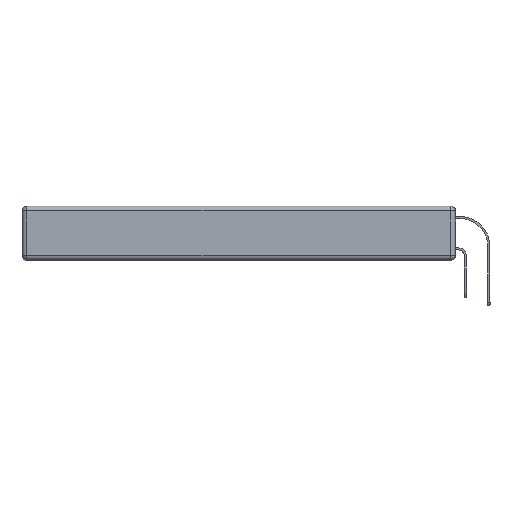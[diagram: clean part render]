
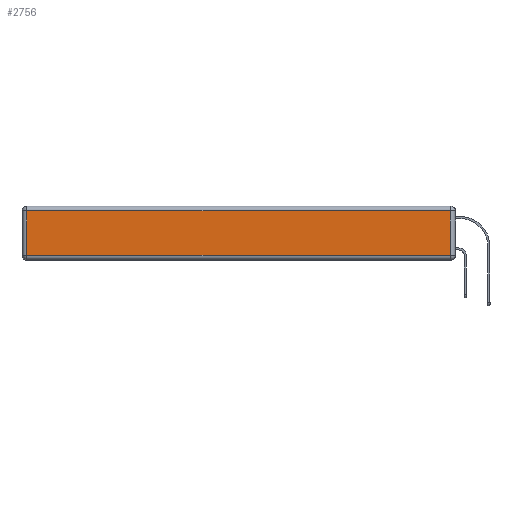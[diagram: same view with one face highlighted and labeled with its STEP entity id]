
A CAD part, left-side view. The second image highlights one B-rep face of the part: STEP entity #2756.
In plain terms, the highlighted planar face has unit normal (-1, 0, 0).
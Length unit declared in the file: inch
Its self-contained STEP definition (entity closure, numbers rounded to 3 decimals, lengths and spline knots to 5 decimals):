
#526 = ORIENTED_EDGE ( 'NONE', *, *, #12476, .T. ) ;
#814 = LINE ( 'NONE', #9463, #4873 ) ;
#867 = VECTOR ( 'NONE', #3666, 39.37008 ) ;
#1168 = CARTESIAN_POINT ( 'NONE',  ( 0., 2.72, -0.03 ) ) ;
#1239 = VERTEX_POINT ( 'NONE', #5424 ) ;
#1809 = CARTESIAN_POINT ( 'NONE',  ( 0., 0., -0.343 ) ) ;
#1946 = DIRECTION ( 'NONE',  ( 0., 0., 1. ) ) ;
#2121 = LINE ( 'NONE', #9834, #4508 ) ;
#2756 = ADVANCED_FACE ( 'NONE', ( #10301 ), #12660, .T. ) ;
#2794 = EDGE_CURVE ( 'NONE', #1239, #9489, #814, .T. ) ;
#2944 = DIRECTION ( 'NONE',  ( -1., 0., 0. ) ) ;
#3602 = CARTESIAN_POINT ( 'NONE',  ( 0., 0., -0.313 ) ) ;
#3666 = DIRECTION ( 'NONE',  ( 0., -1., 0. ) ) ;
#4508 = VECTOR ( 'NONE', #9770, 39.37008 ) ;
#4873 = VECTOR ( 'NONE', #13863, 39.37008 ) ;
#5424 = CARTESIAN_POINT ( 'NONE',  ( 0., 0.03, -0.03 ) ) ;
#5428 = EDGE_CURVE ( 'NONE', #9489, #6274, #2121, .T. ) ;
#6274 = VERTEX_POINT ( 'NONE', #9744 ) ;
#6425 = DIRECTION ( 'NONE',  ( 0., 0., 1. ) ) ;
#7605 = EDGE_CURVE ( 'NONE', #13902, #1239, #11670, .T. ) ;
#8050 = AXIS2_PLACEMENT_3D ( 'NONE', #1809, #2944, #1946 ) ;
#8646 = ORIENTED_EDGE ( 'NONE', *, *, #7605, .T. ) ;
#9463 = CARTESIAN_POINT ( 'NONE',  ( 0., 2.75, -0.03 ) ) ;
#9489 = VERTEX_POINT ( 'NONE', #1168 ) ;
#9744 = CARTESIAN_POINT ( 'NONE',  ( 0., 2.72, -0.313 ) ) ;
#9770 = DIRECTION ( 'NONE',  ( 0., 0., -1. ) ) ;
#9834 = CARTESIAN_POINT ( 'NONE',  ( 0., 2.72, -0.343 ) ) ;
#10301 = FACE_OUTER_BOUND ( 'NONE', #12740, .T. ) ;
#10609 = CARTESIAN_POINT ( 'NONE',  ( 0., 0.03, -0.343 ) ) ;
#11357 = ORIENTED_EDGE ( 'NONE', *, *, #5428, .T. ) ;
#11670 = LINE ( 'NONE', #10609, #13555 ) ;
#12051 = LINE ( 'NONE', #3602, #867 ) ;
#12476 = EDGE_CURVE ( 'NONE', #6274, #13902, #12051, .T. ) ;
#12660 = PLANE ( 'NONE',  #8050 ) ;
#12740 = EDGE_LOOP ( 'NONE', ( #526, #8646, #13056, #11357 ) ) ;
#13056 = ORIENTED_EDGE ( 'NONE', *, *, #2794, .T. ) ;
#13253 = CARTESIAN_POINT ( 'NONE',  ( 0., 0.03, -0.313 ) ) ;
#13555 = VECTOR ( 'NONE', #6425, 39.37008 ) ;
#13863 = DIRECTION ( 'NONE',  ( 0., 1., 0. ) ) ;
#13902 = VERTEX_POINT ( 'NONE', #13253 ) ;
